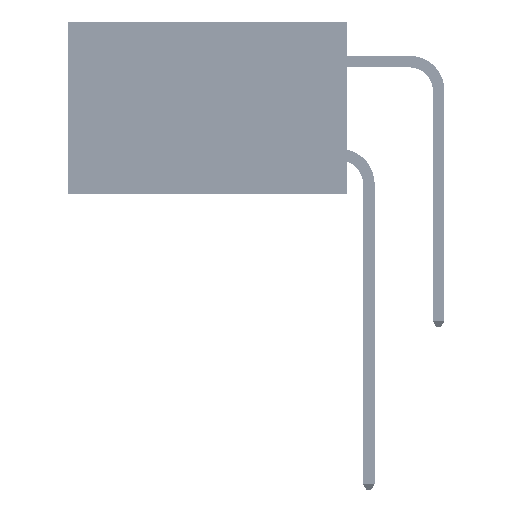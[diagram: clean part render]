
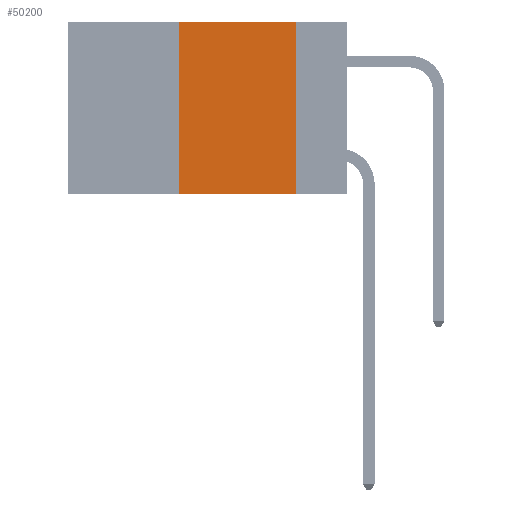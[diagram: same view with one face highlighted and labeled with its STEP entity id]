
A CAD part, left-side view. The second image highlights one B-rep face of the part: STEP entity #50200.
In plain terms, the highlighted planar face has unit normal (-1, 0, 0).
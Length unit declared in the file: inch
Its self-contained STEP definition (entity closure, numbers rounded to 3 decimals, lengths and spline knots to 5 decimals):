
#177 = LINE ( 'NONE', #33404, #49415 ) ;
#533 = LINE ( 'NONE', #16359, #48467 ) ;
#5430 = CARTESIAN_POINT ( 'NONE',  ( 0., 0.11, -0.37 ) ) ;
#5773 = EDGE_CURVE ( 'NONE', #18800, #35759, #533, .T. ) ;
#7295 = DIRECTION ( 'NONE',  ( 0., 0., -1. ) ) ;
#11222 = CARTESIAN_POINT ( 'NONE',  ( 0., 0.6, 0. ) ) ;
#11234 = ORIENTED_EDGE ( 'NONE', *, *, #5773, .F. ) ;
#11521 = VERTEX_POINT ( 'NONE', #19959 ) ;
#12905 = ORIENTED_EDGE ( 'NONE', *, *, #19019, .F. ) ;
#15287 = LINE ( 'NONE', #52149, #31328 ) ;
#16024 = EDGE_LOOP ( 'NONE', ( #11234, #52439, #12905, #47617 ) ) ;
#16359 = CARTESIAN_POINT ( 'NONE',  ( 0., 0.11, 0. ) ) ;
#18800 = VERTEX_POINT ( 'NONE', #34444 ) ;
#19019 = EDGE_CURVE ( 'NONE', #11521, #21487, #15287, .T. ) ;
#19959 = CARTESIAN_POINT ( 'NONE',  ( 0., 0.36, -0.37 ) ) ;
#21013 = VECTOR ( 'NONE', #47283, 39.37008 ) ;
#21487 = VERTEX_POINT ( 'NONE', #29423 ) ;
#27267 = DIRECTION ( 'NONE',  ( 0., 0., 1. ) ) ;
#27840 = PLANE ( 'NONE',  #28615 ) ;
#28615 = AXIS2_PLACEMENT_3D ( 'NONE', #11222, #43942, #7295 ) ;
#29120 = DIRECTION ( 'NONE',  ( 0., -1., 0. ) ) ;
#29423 = CARTESIAN_POINT ( 'NONE',  ( 0., 0.36, 0. ) ) ;
#30682 = CARTESIAN_POINT ( 'NONE',  ( 0., 0.6, 0. ) ) ;
#31328 = VECTOR ( 'NONE', #27267, 39.37008 ) ;
#32928 = EDGE_CURVE ( 'NONE', #11521, #35759, #177, .T. ) ;
#33404 = CARTESIAN_POINT ( 'NONE',  ( 0., 0.6, -0.37 ) ) ;
#34444 = CARTESIAN_POINT ( 'NONE',  ( 0., 0.11, 0. ) ) ;
#34446 = LINE ( 'NONE', #30682, #21013 ) ;
#35759 = VERTEX_POINT ( 'NONE', #5430 ) ;
#41949 = EDGE_CURVE ( 'NONE', #21487, #18800, #34446, .T. ) ;
#43942 = DIRECTION ( 'NONE',  ( 1., 0., 0. ) ) ;
#47283 = DIRECTION ( 'NONE',  ( 0., -1., 0. ) ) ;
#47617 = ORIENTED_EDGE ( 'NONE', *, *, #32928, .T. ) ;
#48110 = FACE_OUTER_BOUND ( 'NONE', #16024, .T. ) ;
#48386 = DIRECTION ( 'NONE',  ( 0., 0., -1. ) ) ;
#48467 = VECTOR ( 'NONE', #48386, 39.37008 ) ;
#49415 = VECTOR ( 'NONE', #29120, 39.37008 ) ;
#50200 = ADVANCED_FACE ( 'NONE', ( #48110 ), #27840, .F. ) ;
#52149 = CARTESIAN_POINT ( 'NONE',  ( 0., 0.36, 0. ) ) ;
#52439 = ORIENTED_EDGE ( 'NONE', *, *, #41949, .F. ) ;
